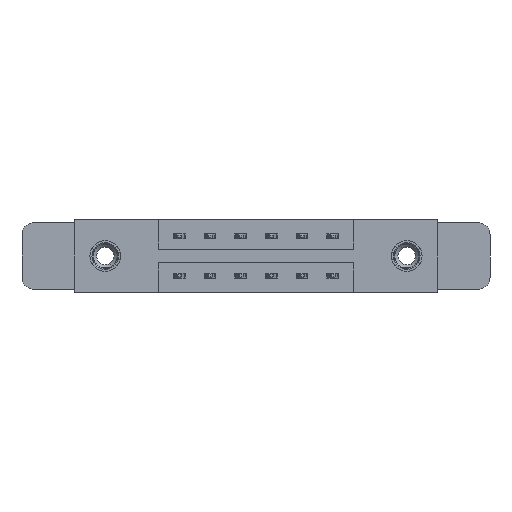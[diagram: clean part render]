
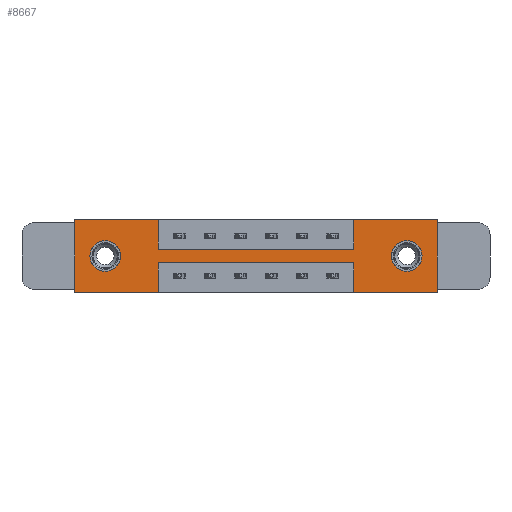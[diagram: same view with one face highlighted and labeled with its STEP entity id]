
A CAD part, front view. The second image highlights one B-rep face of the part: STEP entity #8667.
In plain terms, the highlighted planar face has unit normal (0, -1, 0).
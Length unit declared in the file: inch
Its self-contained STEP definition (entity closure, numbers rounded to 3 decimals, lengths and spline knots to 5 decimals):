
#61 = CARTESIAN_POINT ( 'NONE',  ( 0.425, 0., -0.37 ) ) ;
#113 = VECTOR ( 'NONE', #8391, 39.37008 ) ;
#114 = VERTEX_POINT ( 'NONE', #5414 ) ;
#283 = VERTEX_POINT ( 'NONE', #1068 ) ;
#286 = VERTEX_POINT ( 'NONE', #7563 ) ;
#316 = CARTESIAN_POINT ( 'NONE',  ( 0.425, 0., -0.22 ) ) ;
#331 = CIRCLE ( 'NONE', #5929, 0.078 ) ;
#381 = EDGE_LOOP ( 'NONE', ( #11290, #10544 ) ) ;
#398 = VECTOR ( 'NONE', #11751, 39.37008 ) ;
#442 = EDGE_CURVE ( 'NONE', #5956, #286, #8931, .T. ) ;
#493 = LINE ( 'NONE', #11694, #10663 ) ;
#688 = CARTESIAN_POINT ( 'NONE',  ( 0.425, 0., 0. ) ) ;
#796 = ORIENTED_EDGE ( 'NONE', *, *, #3377, .F. ) ;
#812 = CARTESIAN_POINT ( 'NONE',  ( 0.155, 0., -0.263 ) ) ;
#907 = EDGE_CURVE ( 'NONE', #3988, #5956, #10792, .T. ) ;
#1006 = DIRECTION ( 'NONE',  ( 1., 0., 0. ) ) ;
#1068 = CARTESIAN_POINT ( 'NONE',  ( 1.842, 0., 0. ) ) ;
#1069 = VECTOR ( 'NONE', #3231, 39.37008 ) ;
#1128 = LINE ( 'NONE', #6722, #9704 ) ;
#1167 = CARTESIAN_POINT ( 'NONE',  ( 0., 0., 0. ) ) ;
#1191 = DIRECTION ( 'NONE',  ( 0., 0., -1. ) ) ;
#1255 = CARTESIAN_POINT ( 'NONE',  ( 0., 0., -0.37 ) ) ;
#1488 = VECTOR ( 'NONE', #10951, 39.37008 ) ;
#1534 = VECTOR ( 'NONE', #8698, 39.37008 ) ;
#1672 = DIRECTION ( 'NONE',  ( 0., 0., 1. ) ) ;
#1778 = AXIS2_PLACEMENT_3D ( 'NONE', #11059, #8368, #1672 ) ;
#1834 = VERTEX_POINT ( 'NONE', #8432 ) ;
#1883 = CARTESIAN_POINT ( 'NONE',  ( 1.842, 0., -0.37 ) ) ;
#2110 = EDGE_LOOP ( 'NONE', ( #6972, #9085 ) ) ;
#2550 = CARTESIAN_POINT ( 'NONE',  ( 0., 0., -0.37 ) ) ;
#2553 = LINE ( 'NONE', #61, #113 ) ;
#2683 = EDGE_CURVE ( 'NONE', #3305, #114, #7758, .T. ) ;
#2874 = EDGE_CURVE ( 'NONE', #7618, #7048, #2914, .T. ) ;
#2914 = CIRCLE ( 'NONE', #1778, 0.078 ) ;
#2974 = ORIENTED_EDGE ( 'NONE', *, *, #907, .F. ) ;
#3004 = VECTOR ( 'NONE', #1006, 39.37008 ) ;
#3014 = CIRCLE ( 'NONE', #9299, 0.078 ) ;
#3121 = CARTESIAN_POINT ( 'NONE',  ( 0., 0., -0.37 ) ) ;
#3191 = CARTESIAN_POINT ( 'NONE',  ( 0., 0., 0. ) ) ;
#3218 = EDGE_CURVE ( 'NONE', #4185, #5920, #6568, .T. ) ;
#3231 = DIRECTION ( 'NONE',  ( 0., 0., 1. ) ) ;
#3305 = VERTEX_POINT ( 'NONE', #5544 ) ;
#3377 = EDGE_CURVE ( 'NONE', #114, #10398, #6252, .T. ) ;
#3745 = DIRECTION ( 'NONE',  ( 0., 0., 1. ) ) ;
#3956 = ORIENTED_EDGE ( 'NONE', *, *, #10282, .F. ) ;
#3988 = VERTEX_POINT ( 'NONE', #1883 ) ;
#4068 = VECTOR ( 'NONE', #3745, 39.37008 ) ;
#4080 = VECTOR ( 'NONE', #9081, 39.37008 ) ;
#4125 = DIRECTION ( 'NONE',  ( 0., -1., 0. ) ) ;
#4185 = VERTEX_POINT ( 'NONE', #3121 ) ;
#4193 = CARTESIAN_POINT ( 'NONE',  ( 1.417, 0., -0.37 ) ) ;
#4220 = ORIENTED_EDGE ( 'NONE', *, *, #442, .F. ) ;
#4324 = DIRECTION ( 'NONE',  ( 0., 0., -1. ) ) ;
#4336 = CARTESIAN_POINT ( 'NONE',  ( 1.417, 0., 0. ) ) ;
#4464 = DIRECTION ( 'NONE',  ( 0., 1., 0. ) ) ;
#4511 = DIRECTION ( 'NONE',  ( 0., 0., -1. ) ) ;
#5060 = LINE ( 'NONE', #1255, #1534 ) ;
#5414 = CARTESIAN_POINT ( 'NONE',  ( 1.417, 0., -0.15 ) ) ;
#5447 = FACE_OUTER_BOUND ( 'NONE', #7467, .T. ) ;
#5544 = CARTESIAN_POINT ( 'NONE',  ( 0.425, 0., -0.15 ) ) ;
#5665 = AXIS2_PLACEMENT_3D ( 'NONE', #7003, #4125, #10728 ) ;
#5699 = EDGE_CURVE ( 'NONE', #5934, #8212, #2553, .T. ) ;
#5920 = VERTEX_POINT ( 'NONE', #3191 ) ;
#5929 = AXIS2_PLACEMENT_3D ( 'NONE', #10404, #9441, #1191 ) ;
#5934 = VERTEX_POINT ( 'NONE', #316 ) ;
#5956 = VERTEX_POINT ( 'NONE', #6990 ) ;
#6138 = EDGE_CURVE ( 'NONE', #1834, #6153, #3014, .T. ) ;
#6153 = VERTEX_POINT ( 'NONE', #11787 ) ;
#6206 = VERTEX_POINT ( 'NONE', #688 ) ;
#6238 = EDGE_CURVE ( 'NONE', #5920, #6206, #11560, .T. ) ;
#6252 = LINE ( 'NONE', #8310, #4068 ) ;
#6275 = VECTOR ( 'NONE', #7054, 39.37008 ) ;
#6568 = LINE ( 'NONE', #11726, #4080 ) ;
#6722 = CARTESIAN_POINT ( 'NONE',  ( 0.425, 0., -0.22 ) ) ;
#6725 = CARTESIAN_POINT ( 'NONE',  ( 0.425, 0., -0.15 ) ) ;
#6832 = ORIENTED_EDGE ( 'NONE', *, *, #3218, .F. ) ;
#6972 = ORIENTED_EDGE ( 'NONE', *, *, #11462, .T. ) ;
#6990 = CARTESIAN_POINT ( 'NONE',  ( 1.417, 0., -0.37 ) ) ;
#7003 = CARTESIAN_POINT ( 'NONE',  ( 0., 0., -0.37 ) ) ;
#7048 = VERTEX_POINT ( 'NONE', #10245 ) ;
#7054 = DIRECTION ( 'NONE',  ( 1., 0., 0. ) ) ;
#7107 = ORIENTED_EDGE ( 'NONE', *, *, #8506, .F. ) ;
#7158 = ORIENTED_EDGE ( 'NONE', *, *, #7950, .F. ) ;
#7245 = CARTESIAN_POINT ( 'NONE',  ( 0.425, 0., 0. ) ) ;
#7402 = ORIENTED_EDGE ( 'NONE', *, *, #5699, .F. ) ;
#7467 = EDGE_LOOP ( 'NONE', ( #7402, #8381, #4220, #2974, #9276, #7107, #796, #11540, #7158, #8410, #6832, #3956 ) ) ;
#7546 = CARTESIAN_POINT ( 'NONE',  ( 0., 0., 0. ) ) ;
#7563 = CARTESIAN_POINT ( 'NONE',  ( 1.417, 0., -0.22 ) ) ;
#7618 = VERTEX_POINT ( 'NONE', #812 ) ;
#7758 = LINE ( 'NONE', #6725, #6275 ) ;
#7828 = DIRECTION ( 'NONE',  ( 1., 0., 0. ) ) ;
#7903 = PLANE ( 'NONE',  #5665 ) ;
#7935 = CARTESIAN_POINT ( 'NONE',  ( 0.155, 0., -0.185 ) ) ;
#7950 = EDGE_CURVE ( 'NONE', #6206, #3305, #11117, .T. ) ;
#7954 = FACE_BOUND ( 'NONE', #381, .T. ) ;
#8212 = VERTEX_POINT ( 'NONE', #10010 ) ;
#8310 = CARTESIAN_POINT ( 'NONE',  ( 1.417, 0., 0. ) ) ;
#8329 = CIRCLE ( 'NONE', #10713, 0.078 ) ;
#8357 = LINE ( 'NONE', #1167, #10083 ) ;
#8368 = DIRECTION ( 'NONE',  ( 0., 1., 0. ) ) ;
#8381 = ORIENTED_EDGE ( 'NONE', *, *, #10108, .F. ) ;
#8391 = DIRECTION ( 'NONE',  ( 0., 0., -1. ) ) ;
#8410 = ORIENTED_EDGE ( 'NONE', *, *, #6238, .F. ) ;
#8411 = DIRECTION ( 'NONE',  ( -1., 0., 0. ) ) ;
#8432 = CARTESIAN_POINT ( 'NONE',  ( 1.687, 0., -0.263 ) ) ;
#8506 = EDGE_CURVE ( 'NONE', #10398, #283, #8357, .T. ) ;
#8667 = ADVANCED_FACE ( 'NONE', ( #8945, #7954, #5447 ), #7903, .T. ) ;
#8698 = DIRECTION ( 'NONE',  ( -1., 0., 0. ) ) ;
#8726 = DIRECTION ( 'NONE',  ( 0., 0., 1. ) ) ;
#8795 = EDGE_CURVE ( 'NONE', #283, #3988, #493, .T. ) ;
#8931 = LINE ( 'NONE', #4193, #1069 ) ;
#8945 = FACE_BOUND ( 'NONE', #2110, .T. ) ;
#9081 = DIRECTION ( 'NONE',  ( 0., 0., 1. ) ) ;
#9085 = ORIENTED_EDGE ( 'NONE', *, *, #6138, .T. ) ;
#9276 = ORIENTED_EDGE ( 'NONE', *, *, #8795, .F. ) ;
#9299 = AXIS2_PLACEMENT_3D ( 'NONE', #10869, #4464, #4511 ) ;
#9441 = DIRECTION ( 'NONE',  ( 0., 1., 0. ) ) ;
#9704 = VECTOR ( 'NONE', #8411, 39.37008 ) ;
#10010 = CARTESIAN_POINT ( 'NONE',  ( 0.425, 0., -0.37 ) ) ;
#10083 = VECTOR ( 'NONE', #7828, 39.37008 ) ;
#10108 = EDGE_CURVE ( 'NONE', #286, #5934, #1128, .T. ) ;
#10245 = CARTESIAN_POINT ( 'NONE',  ( 0.155, 0., -0.107 ) ) ;
#10282 = EDGE_CURVE ( 'NONE', #8212, #4185, #5060, .T. ) ;
#10398 = VERTEX_POINT ( 'NONE', #4336 ) ;
#10404 = CARTESIAN_POINT ( 'NONE',  ( 1.687, 0., -0.185 ) ) ;
#10544 = ORIENTED_EDGE ( 'NONE', *, *, #2874, .T. ) ;
#10663 = VECTOR ( 'NONE', #4324, 39.37008 ) ;
#10713 = AXIS2_PLACEMENT_3D ( 'NONE', #7935, #11508, #8726 ) ;
#10728 = DIRECTION ( 'NONE',  ( 0., 0., -1. ) ) ;
#10792 = LINE ( 'NONE', #2550, #1488 ) ;
#10869 = CARTESIAN_POINT ( 'NONE',  ( 1.687, 0., -0.185 ) ) ;
#10945 = EDGE_CURVE ( 'NONE', #7048, #7618, #8329, .T. ) ;
#10951 = DIRECTION ( 'NONE',  ( -1., 0., 0. ) ) ;
#11059 = CARTESIAN_POINT ( 'NONE',  ( 0.155, 0., -0.185 ) ) ;
#11117 = LINE ( 'NONE', #7245, #398 ) ;
#11290 = ORIENTED_EDGE ( 'NONE', *, *, #10945, .T. ) ;
#11462 = EDGE_CURVE ( 'NONE', #6153, #1834, #331, .T. ) ;
#11508 = DIRECTION ( 'NONE',  ( 0., 1., 0. ) ) ;
#11540 = ORIENTED_EDGE ( 'NONE', *, *, #2683, .F. ) ;
#11560 = LINE ( 'NONE', #7546, #3004 ) ;
#11694 = CARTESIAN_POINT ( 'NONE',  ( 1.842, 0., 0. ) ) ;
#11726 = CARTESIAN_POINT ( 'NONE',  ( 0., 0., 0. ) ) ;
#11751 = DIRECTION ( 'NONE',  ( 0., 0., -1. ) ) ;
#11787 = CARTESIAN_POINT ( 'NONE',  ( 1.687, 0., -0.107 ) ) ;
